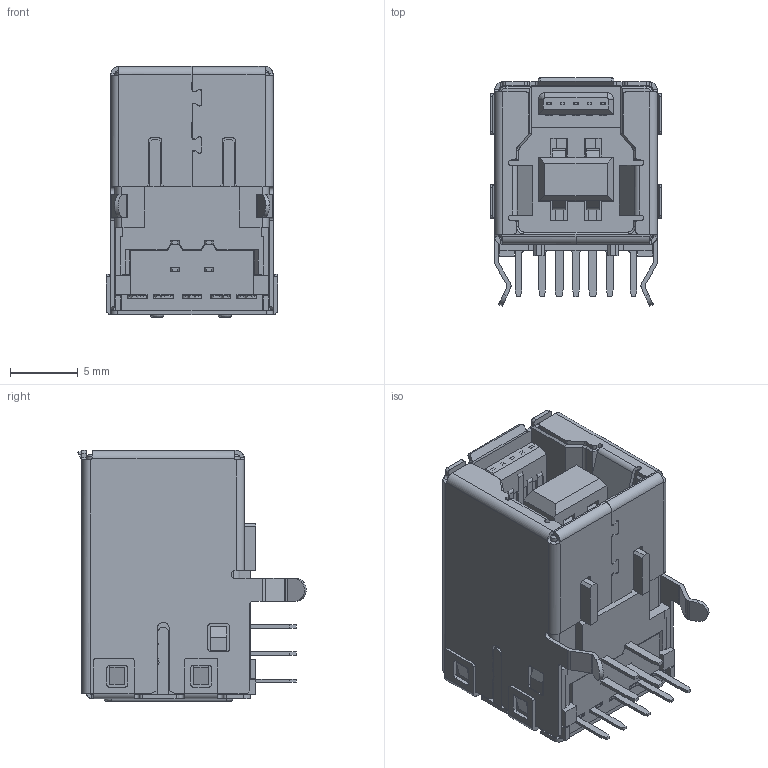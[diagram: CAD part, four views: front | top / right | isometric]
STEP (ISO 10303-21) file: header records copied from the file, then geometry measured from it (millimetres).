
FILE_DESCRIPTION (( 'STEP AP214' ), '1' );
FILE_NAME ('690P209-12C-021.STEP', '2021-01-14T21:14:15', ( '' ), ( '' ), 'SwSTEP 2.0', 'SolidWorks 2020', '' );
FILE_SCHEMA (( 'AUTOMOTIVE_DESIGN' ));
Length unit declared in the file: millimetre
Products named in the file (13): Contact9 690P209-X2C-02X; Contact8 690P209-X2C-02X; Insulator1 690P209-X2C-02X_Black; Contact1 690P209-X2C-02X; Contact6 690P209-X2C-02X; Shell2 690P209-X2C-02X; Contact5 690P209-X2C-02X; Contact2 690P209-X2C-02X; Insulator2 690P209-X2C-02X_Black; Shell 690P209-X2C-02X; Insulator3 690P209-X2C-02X_Black; 690P209-12C-021; Contact7 690P209-X2C-02X
Assembly tree (14 placements, depth 2):
  690P209-12C-021
    Shell 690P209-X2C-02X
    Insulator1 690P209-X2C-02X_Black
    Contact7 690P209-X2C-02X
    Insulator2 690P209-X2C-02X_Black
    Contact6 690P209-X2C-02X
    Contact5 690P209-X2C-02X
    Contact8 690P209-X2C-02X
    Contact9 690P209-X2C-02X
    Insulator3 690P209-X2C-02X_Black
    Shell2 690P209-X2C-02X
    Contact1 690P209-X2C-02X  x2
    Contact2 690P209-X2C-02X  x2
Bounding box: 12.7 x 16.88 x 18.55 mm (x, y, z)
Volume: 1478.7 mm3; surface area: 5371.2 mm2
Topology: 14 solids, 14 shells, 1460 faces, 4095 edges, 2662 vertices
Faces by surface type: plane 1032, cylinder 354, bspline 60, cone 14
Entity records: 45489 total; most frequent: CARTESIAN_POINT 11349, ORIENTED_EDGE 7408, DIRECTION 6345, EDGE_CURVE 3704, LINE 2909, VECTOR 2909, VERTEX_POINT 2404, AXIS2_PLACEMENT_3D 1718
